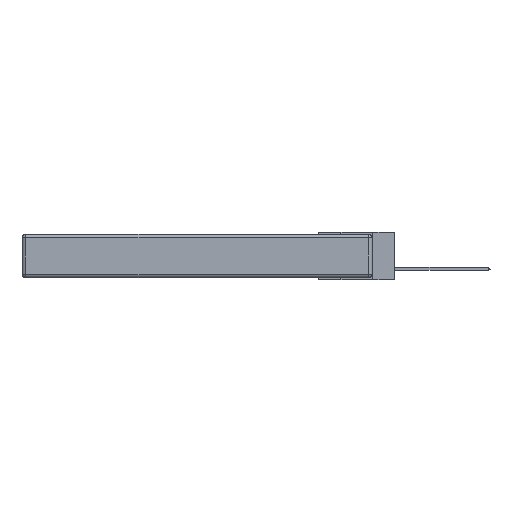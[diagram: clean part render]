
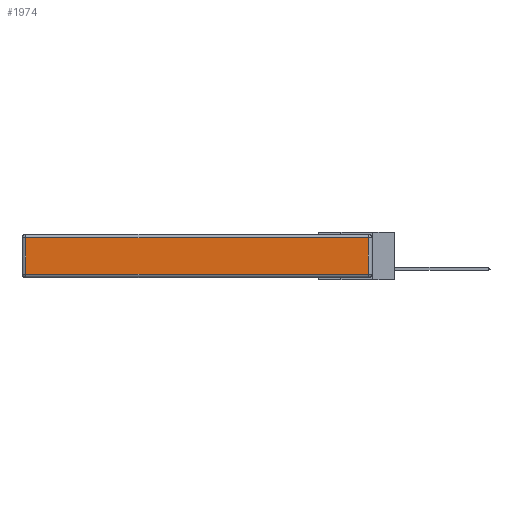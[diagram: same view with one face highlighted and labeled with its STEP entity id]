
A CAD part, left-side view. The second image highlights one B-rep face of the part: STEP entity #1974.
In plain terms, the highlighted planar face has unit normal (-1, 0, 0).
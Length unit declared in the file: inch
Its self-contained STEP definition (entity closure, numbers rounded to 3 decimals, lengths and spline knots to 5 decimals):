
#539 = ORIENTED_EDGE ( 'NONE', *, *, #18774, .T. ) ;
#1045 = ORIENTED_EDGE ( 'NONE', *, *, #12349, .T. ) ;
#1974 = ADVANCED_FACE ( 'NONE', ( #15223 ), #7573, .T. ) ;
#3390 = DIRECTION ( 'NONE',  ( 0., 1., 0. ) ) ;
#3646 = CARTESIAN_POINT ( 'NONE',  ( 0., 0.03, -0.343 ) ) ;
#4546 = CARTESIAN_POINT ( 'NONE',  ( 0., 0., -0.313 ) ) ;
#4620 = VERTEX_POINT ( 'NONE', #20238 ) ;
#4971 = EDGE_CURVE ( 'NONE', #7643, #19053, #9094, .T. ) ;
#5815 = VECTOR ( 'NONE', #19574, 39.37008 ) ;
#6016 = LINE ( 'NONE', #11590, #12256 ) ;
#6726 = CARTESIAN_POINT ( 'NONE',  ( 0., 2.75, -0.03 ) ) ;
#7573 = PLANE ( 'NONE',  #9031 ) ;
#7608 = ORIENTED_EDGE ( 'NONE', *, *, #4971, .T. ) ;
#7643 = VERTEX_POINT ( 'NONE', #14158 ) ;
#9031 = AXIS2_PLACEMENT_3D ( 'NONE', #12424, #15583, #12233 ) ;
#9094 = LINE ( 'NONE', #4546, #15348 ) ;
#9640 = CARTESIAN_POINT ( 'NONE',  ( 0., 2.72, -0.03 ) ) ;
#10723 = LINE ( 'NONE', #6726, #19194 ) ;
#11590 = CARTESIAN_POINT ( 'NONE',  ( 0., 2.72, -0.343 ) ) ;
#11931 = VERTEX_POINT ( 'NONE', #9640 ) ;
#12233 = DIRECTION ( 'NONE',  ( 0., 0., 1. ) ) ;
#12256 = VECTOR ( 'NONE', #16814, 39.37008 ) ;
#12349 = EDGE_CURVE ( 'NONE', #11931, #7643, #6016, .T. ) ;
#12424 = CARTESIAN_POINT ( 'NONE',  ( 0., 0., -0.343 ) ) ;
#14022 = ORIENTED_EDGE ( 'NONE', *, *, #16868, .T. ) ;
#14158 = CARTESIAN_POINT ( 'NONE',  ( 0., 2.72, -0.313 ) ) ;
#15223 = FACE_OUTER_BOUND ( 'NONE', #17205, .T. ) ;
#15348 = VECTOR ( 'NONE', #19174, 39.37008 ) ;
#15583 = DIRECTION ( 'NONE',  ( -1., 0., 0. ) ) ;
#16545 = CARTESIAN_POINT ( 'NONE',  ( 0., 0.03, -0.313 ) ) ;
#16814 = DIRECTION ( 'NONE',  ( 0., 0., -1. ) ) ;
#16868 = EDGE_CURVE ( 'NONE', #19053, #4620, #18755, .T. ) ;
#17205 = EDGE_LOOP ( 'NONE', ( #7608, #14022, #539, #1045 ) ) ;
#18755 = LINE ( 'NONE', #3646, #5815 ) ;
#18774 = EDGE_CURVE ( 'NONE', #4620, #11931, #10723, .T. ) ;
#19053 = VERTEX_POINT ( 'NONE', #16545 ) ;
#19174 = DIRECTION ( 'NONE',  ( 0., -1., 0. ) ) ;
#19194 = VECTOR ( 'NONE', #3390, 39.37008 ) ;
#19574 = DIRECTION ( 'NONE',  ( 0., 0., 1. ) ) ;
#20238 = CARTESIAN_POINT ( 'NONE',  ( 0., 0.03, -0.03 ) ) ;
